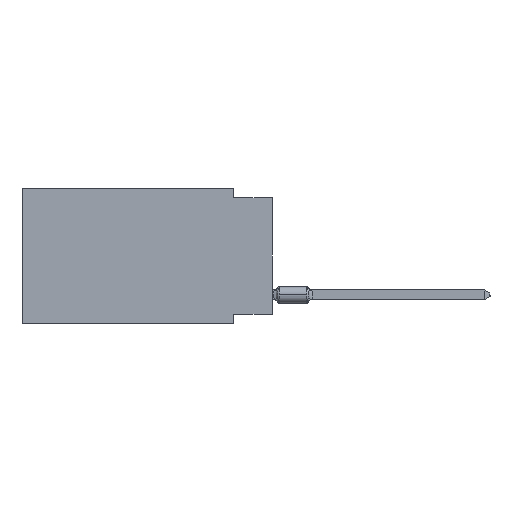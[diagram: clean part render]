
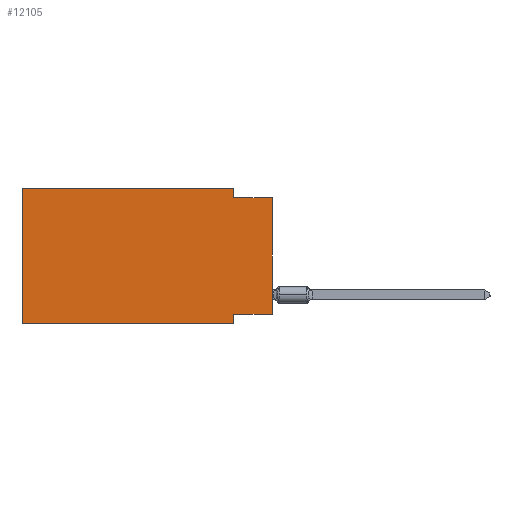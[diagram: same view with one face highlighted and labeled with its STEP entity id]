
A CAD part, left-side view. The second image highlights one B-rep face of the part: STEP entity #12105.
In plain terms, the highlighted planar face has unit normal (-1, 0, 0).
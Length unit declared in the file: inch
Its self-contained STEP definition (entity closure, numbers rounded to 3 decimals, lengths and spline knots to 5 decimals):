
#154 = CARTESIAN_POINT ( 'NONE',  ( 0., 0.645, 0. ) ) ;
#911 = LINE ( 'NONE', #46483, #5216 ) ;
#1061 = DIRECTION ( 'NONE',  ( 0., -1., 0. ) ) ;
#1611 = CARTESIAN_POINT ( 'NONE',  ( 0., 0.1, -0.35 ) ) ;
#2386 = ORIENTED_EDGE ( 'NONE', *, *, #24776, .F. ) ;
#2766 = AXIS2_PLACEMENT_3D ( 'NONE', #154, #39062, #43146 ) ;
#2768 = LINE ( 'NONE', #22487, #46175 ) ;
#3774 = PLANE ( 'NONE',  #2766 ) ;
#5216 = VECTOR ( 'NONE', #11446, 39.37008 ) ;
#5645 = CARTESIAN_POINT ( 'NONE',  ( 0., 0.1, 0. ) ) ;
#9007 = LINE ( 'NONE', #47619, #20980 ) ;
#10047 = VERTEX_POINT ( 'NONE', #5645 ) ;
#11446 = DIRECTION ( 'NONE',  ( 0., -1., 0. ) ) ;
#12105 = ADVANCED_FACE ( 'NONE', ( #35474 ), #3774, .F. ) ;
#12198 = EDGE_CURVE ( 'NONE', #41436, #33950, #911, .T. ) ;
#12792 = VECTOR ( 'NONE', #13719, 39.37008 ) ;
#13719 = DIRECTION ( 'NONE',  ( 0., 1., 0. ) ) ;
#14196 = CARTESIAN_POINT ( 'NONE',  ( 0., 0., 0. ) ) ;
#14590 = VERTEX_POINT ( 'NONE', #27372 ) ;
#17379 = CARTESIAN_POINT ( 'NONE',  ( 0., 0.645, -0.35 ) ) ;
#17407 = EDGE_CURVE ( 'NONE', #23377, #44367, #21856, .T. ) ;
#17766 = ORIENTED_EDGE ( 'NONE', *, *, #17407, .F. ) ;
#20980 = VECTOR ( 'NONE', #1061, 39.37008 ) ;
#21856 = LINE ( 'NONE', #1611, #43549 ) ;
#22487 = CARTESIAN_POINT ( 'NONE',  ( 0., 0.645, 0. ) ) ;
#22958 = CARTESIAN_POINT ( 'NONE',  ( 0., 0.1, -0.325 ) ) ;
#23377 = VERTEX_POINT ( 'NONE', #22958 ) ;
#24515 = VECTOR ( 'NONE', #30063, 39.37008 ) ;
#24646 = ORIENTED_EDGE ( 'NONE', *, *, #48068, .T. ) ;
#24776 = EDGE_CURVE ( 'NONE', #49753, #23377, #33397, .T. ) ;
#25196 = ORIENTED_EDGE ( 'NONE', *, *, #45349, .F. ) ;
#27372 = CARTESIAN_POINT ( 'NONE',  ( 0., 0.645, 0. ) ) ;
#28193 = CARTESIAN_POINT ( 'NONE',  ( 0., 0.1, -0.025 ) ) ;
#28280 = VECTOR ( 'NONE', #47800, 39.37008 ) ;
#29296 = EDGE_LOOP ( 'NONE', ( #24646, #39708, #49154, #32441, #25196, #42542, #17766, #2386 ) ) ;
#29758 = DIRECTION ( 'NONE',  ( 0., 0., -1. ) ) ;
#29791 = DIRECTION ( 'NONE',  ( 0., 0., 1. ) ) ;
#30063 = DIRECTION ( 'NONE',  ( 0., 0., -1. ) ) ;
#31084 = CARTESIAN_POINT ( 'NONE',  ( 0., 0.645, -0.35 ) ) ;
#31761 = VERTEX_POINT ( 'NONE', #31084 ) ;
#32441 = ORIENTED_EDGE ( 'NONE', *, *, #46409, .F. ) ;
#33397 = LINE ( 'NONE', #45404, #12792 ) ;
#33950 = VERTEX_POINT ( 'NONE', #40985 ) ;
#34636 = LINE ( 'NONE', #45391, #24515 ) ;
#35309 = CARTESIAN_POINT ( 'NONE',  ( 0., 0., -0.325 ) ) ;
#35474 = FACE_OUTER_BOUND ( 'NONE', #29296, .T. ) ;
#35799 = LINE ( 'NONE', #17379, #28280 ) ;
#39062 = DIRECTION ( 'NONE',  ( 1., 0., 0. ) ) ;
#39708 = ORIENTED_EDGE ( 'NONE', *, *, #12198, .F. ) ;
#40985 = CARTESIAN_POINT ( 'NONE',  ( 0., 0., -0.025 ) ) ;
#41436 = VERTEX_POINT ( 'NONE', #28193 ) ;
#41658 = DIRECTION ( 'NONE',  ( 0., 0., 1. ) ) ;
#42542 = ORIENTED_EDGE ( 'NONE', *, *, #44003, .T. ) ;
#43146 = DIRECTION ( 'NONE',  ( 0., 0., -1. ) ) ;
#43549 = VECTOR ( 'NONE', #29758, 39.37008 ) ;
#44003 = EDGE_CURVE ( 'NONE', #31761, #44367, #35799, .T. ) ;
#44367 = VERTEX_POINT ( 'NONE', #44402 ) ;
#44402 = CARTESIAN_POINT ( 'NONE',  ( 0., 0.1, -0.35 ) ) ;
#45349 = EDGE_CURVE ( 'NONE', #31761, #14590, #2768, .T. ) ;
#45391 = CARTESIAN_POINT ( 'NONE',  ( 0., 0.1, 0. ) ) ;
#45404 = CARTESIAN_POINT ( 'NONE',  ( 0., 0., -0.325 ) ) ;
#46175 = VECTOR ( 'NONE', #41658, 39.37008 ) ;
#46409 = EDGE_CURVE ( 'NONE', #14590, #10047, #9007, .T. ) ;
#46483 = CARTESIAN_POINT ( 'NONE',  ( 0., 0., -0.025 ) ) ;
#47619 = CARTESIAN_POINT ( 'NONE',  ( 0., 0.645, 0. ) ) ;
#47800 = DIRECTION ( 'NONE',  ( 0., -1., 0. ) ) ;
#48068 = EDGE_CURVE ( 'NONE', #49753, #33950, #49963, .T. ) ;
#49154 = ORIENTED_EDGE ( 'NONE', *, *, #49247, .F. ) ;
#49247 = EDGE_CURVE ( 'NONE', #10047, #41436, #34636, .T. ) ;
#49753 = VERTEX_POINT ( 'NONE', #35309 ) ;
#49963 = LINE ( 'NONE', #14196, #50506 ) ;
#50506 = VECTOR ( 'NONE', #29791, 39.37008 ) ;
